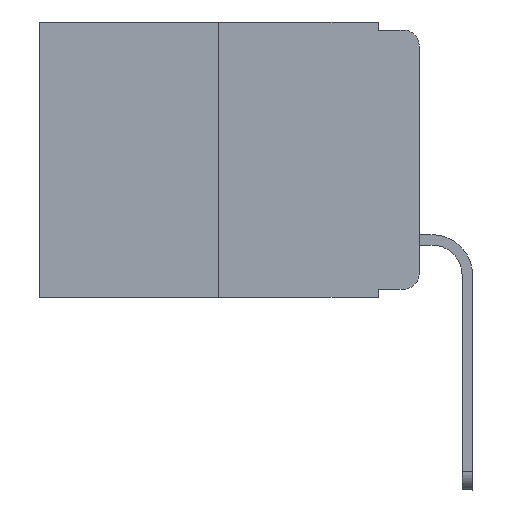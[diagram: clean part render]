
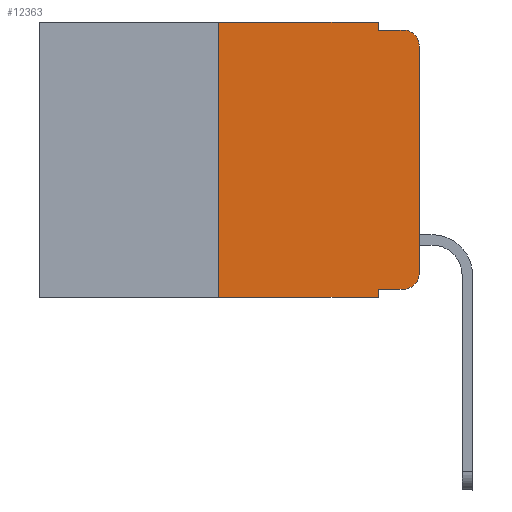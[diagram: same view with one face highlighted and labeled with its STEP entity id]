
A CAD part, left-side view. The second image highlights one B-rep face of the part: STEP entity #12363.
In plain terms, the highlighted planar face has unit normal (-1, 0, 0).
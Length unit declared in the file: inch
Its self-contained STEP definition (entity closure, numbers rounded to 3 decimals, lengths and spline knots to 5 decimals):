
#1009 = DIRECTION ( 'NONE',  ( 0., 0., -1. ) ) ;
#1093 = VERTEX_POINT ( 'NONE', #8850 ) ;
#1252 = CARTESIAN_POINT ( 'NONE',  ( 0., 0.02, -0.03 ) ) ;
#1360 = VERTEX_POINT ( 'NONE', #4169 ) ;
#1515 = CARTESIAN_POINT ( 'NONE',  ( 0., 0.473, 0. ) ) ;
#1548 = VERTEX_POINT ( 'NONE', #12267 ) ;
#1584 = ORIENTED_EDGE ( 'NONE', *, *, #15114, .T. ) ;
#1798 = AXIS2_PLACEMENT_3D ( 'NONE', #15318, #15205, #3770 ) ;
#1992 = AXIS2_PLACEMENT_3D ( 'NONE', #13893, #11682, #8113 ) ;
#2446 = PLANE ( 'NONE',  #1992 ) ;
#2861 = VECTOR ( 'NONE', #1009, 39.37008 ) ;
#3471 = CARTESIAN_POINT ( 'NONE',  ( 0., 0., -0.313 ) ) ;
#3729 = VECTOR ( 'NONE', #5900, 39.37008 ) ;
#3770 = DIRECTION ( 'NONE',  ( 0., 0., -1. ) ) ;
#4013 = VERTEX_POINT ( 'NONE', #10336 ) ;
#4169 = CARTESIAN_POINT ( 'NONE',  ( 0., 0.02, -0.333 ) ) ;
#4342 = ORIENTED_EDGE ( 'NONE', *, *, #5996, .T. ) ;
#4683 = DIRECTION ( 'NONE',  ( 0., -1., 0. ) ) ;
#5440 = DIRECTION ( 'NONE',  ( 0., -1., 0. ) ) ;
#5648 = ORIENTED_EDGE ( 'NONE', *, *, #11851, .T. ) ;
#5660 = CARTESIAN_POINT ( 'NONE',  ( 0., 0.051, -0.01 ) ) ;
#5900 = DIRECTION ( 'NONE',  ( 0., -1., 0. ) ) ;
#5996 = EDGE_CURVE ( 'NONE', #23332, #20307, #9051, .T. ) ;
#6003 = LINE ( 'NONE', #13510, #22603 ) ;
#6145 = FACE_OUTER_BOUND ( 'NONE', #8439, .T. ) ;
#6798 = VECTOR ( 'NONE', #5440, 39.37008 ) ;
#7043 = VERTEX_POINT ( 'NONE', #9479 ) ;
#8113 = DIRECTION ( 'NONE',  ( 0., 0., -1. ) ) ;
#8147 = EDGE_CURVE ( 'NONE', #11544, #4013, #18633, .T. ) ;
#8359 = DIRECTION ( 'NONE',  ( 0., 0., 1. ) ) ;
#8439 = EDGE_LOOP ( 'NONE', ( #4342, #1584, #19563, #10060, #21452, #21818, #5648, #20140, #16598, #17227 ) ) ;
#8486 = EDGE_CURVE ( 'NONE', #4013, #1093, #16140, .T. ) ;
#8601 = LINE ( 'NONE', #23770, #15406 ) ;
#8628 = DIRECTION ( 'NONE',  ( 0., 0., -1. ) ) ;
#8850 = CARTESIAN_POINT ( 'NONE',  ( 0., 0.051, -0.01 ) ) ;
#9051 = LINE ( 'NONE', #24102, #14779 ) ;
#9479 = CARTESIAN_POINT ( 'NONE',  ( 0., 0.051, -0.333 ) ) ;
#10060 = ORIENTED_EDGE ( 'NONE', *, *, #8486, .F. ) ;
#10080 = EDGE_CURVE ( 'NONE', #20816, #11544, #18224, .T. ) ;
#10336 = CARTESIAN_POINT ( 'NONE',  ( 0., 0.051, 0. ) ) ;
#10409 = VECTOR ( 'NONE', #4683, 39.37008 ) ;
#10893 = EDGE_CURVE ( 'NONE', #1360, #23332, #23056, .T. ) ;
#11140 = DIRECTION ( 'NONE',  ( 0., 0., 1. ) ) ;
#11310 = LINE ( 'NONE', #5660, #3729 ) ;
#11544 = VERTEX_POINT ( 'NONE', #12450 ) ;
#11682 = DIRECTION ( 'NONE',  ( 1., 0., 0. ) ) ;
#11851 = EDGE_CURVE ( 'NONE', #20816, #1548, #14034, .T. ) ;
#12077 = CARTESIAN_POINT ( 'NONE',  ( 0., 0.02, -0.01 ) ) ;
#12267 = CARTESIAN_POINT ( 'NONE',  ( 0., 0.051, -0.343 ) ) ;
#12363 = ADVANCED_FACE ( 'NONE', ( #6145 ), #2446, .F. ) ;
#12450 = CARTESIAN_POINT ( 'NONE',  ( 0., 0.25, 0. ) ) ;
#13510 = CARTESIAN_POINT ( 'NONE',  ( 0., 0.051, 0. ) ) ;
#13893 = CARTESIAN_POINT ( 'NONE',  ( 0., 0.473, 0. ) ) ;
#14034 = LINE ( 'NONE', #21581, #10409 ) ;
#14779 = VECTOR ( 'NONE', #11140, 39.37008 ) ;
#15109 = DIRECTION ( 'NONE',  ( 0., -1., 0. ) ) ;
#15114 = EDGE_CURVE ( 'NONE', #20307, #20715, #20226, .T. ) ;
#15205 = DIRECTION ( 'NONE',  ( -1., 0., 0. ) ) ;
#15289 = CARTESIAN_POINT ( 'NONE',  ( 0., 0., -0.03 ) ) ;
#15318 = CARTESIAN_POINT ( 'NONE',  ( 0., 0.02, -0.313 ) ) ;
#15406 = VECTOR ( 'NONE', #15109, 39.37008 ) ;
#15423 = EDGE_CURVE ( 'NONE', #7043, #1548, #6003, .T. ) ;
#15489 = AXIS2_PLACEMENT_3D ( 'NONE', #1252, #16034, #8628 ) ;
#16026 = CARTESIAN_POINT ( 'NONE',  ( 0., 0.25, -0.343 ) ) ;
#16034 = DIRECTION ( 'NONE',  ( -1., 0., 0. ) ) ;
#16140 = LINE ( 'NONE', #21596, #2861 ) ;
#16598 = ORIENTED_EDGE ( 'NONE', *, *, #22456, .T. ) ;
#17227 = ORIENTED_EDGE ( 'NONE', *, *, #10893, .T. ) ;
#17564 = EDGE_CURVE ( 'NONE', #1093, #20715, #11310, .T. ) ;
#18224 = LINE ( 'NONE', #23648, #22966 ) ;
#18633 = LINE ( 'NONE', #1515, #6798 ) ;
#19563 = ORIENTED_EDGE ( 'NONE', *, *, #17564, .F. ) ;
#20140 = ORIENTED_EDGE ( 'NONE', *, *, #15423, .F. ) ;
#20226 = CIRCLE ( 'NONE', #15489, 0.02 ) ;
#20307 = VERTEX_POINT ( 'NONE', #15289 ) ;
#20715 = VERTEX_POINT ( 'NONE', #12077 ) ;
#20816 = VERTEX_POINT ( 'NONE', #16026 ) ;
#21452 = ORIENTED_EDGE ( 'NONE', *, *, #8147, .F. ) ;
#21581 = CARTESIAN_POINT ( 'NONE',  ( 0., 0.473, -0.343 ) ) ;
#21596 = CARTESIAN_POINT ( 'NONE',  ( 0., 0.051, 0. ) ) ;
#21818 = ORIENTED_EDGE ( 'NONE', *, *, #10080, .F. ) ;
#22456 = EDGE_CURVE ( 'NONE', #7043, #1360, #8601, .T. ) ;
#22603 = VECTOR ( 'NONE', #23023, 39.37008 ) ;
#22966 = VECTOR ( 'NONE', #8359, 39.37008 ) ;
#23023 = DIRECTION ( 'NONE',  ( 0., 0., -1. ) ) ;
#23056 = CIRCLE ( 'NONE', #1798, 0.02 ) ;
#23332 = VERTEX_POINT ( 'NONE', #3471 ) ;
#23648 = CARTESIAN_POINT ( 'NONE',  ( 0., 0.25, 0. ) ) ;
#23770 = CARTESIAN_POINT ( 'NONE',  ( 0., 0.051, -0.333 ) ) ;
#24102 = CARTESIAN_POINT ( 'NONE',  ( 0., 0., 0. ) ) ;
